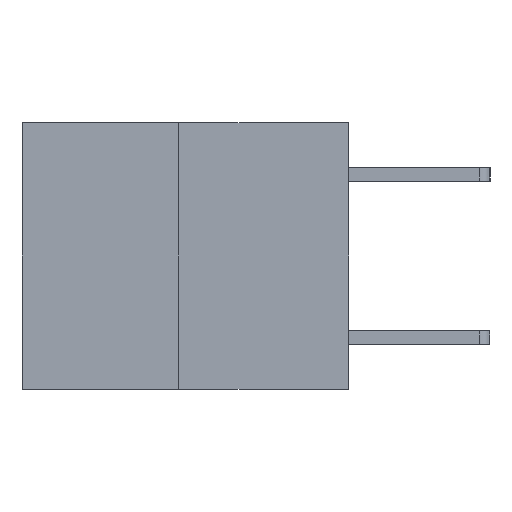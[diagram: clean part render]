
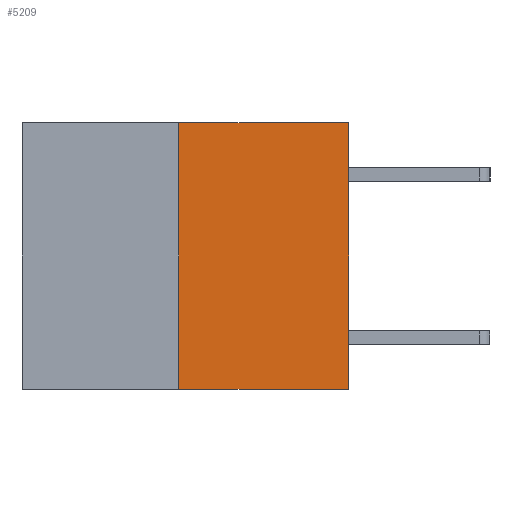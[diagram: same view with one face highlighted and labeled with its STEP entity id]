
A CAD part, left-side view. The second image highlights one B-rep face of the part: STEP entity #5209.
In plain terms, the highlighted planar face has unit normal (-1, 0, 0).
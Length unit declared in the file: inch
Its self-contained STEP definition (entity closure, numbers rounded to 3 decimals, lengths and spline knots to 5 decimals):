
#33 = ORIENTED_EDGE ( 'NONE', *, *, #299, .F. ) ;
#299 = EDGE_CURVE ( 'NONE', #6227, #8768, #3671, .T. ) ;
#565 = CARTESIAN_POINT ( 'NONE',  ( 0., 0., -0.49 ) ) ;
#566 = CARTESIAN_POINT ( 'NONE',  ( 0., 0., 0. ) ) ;
#585 = LINE ( 'NONE', #2959, #3231 ) ;
#1398 = CARTESIAN_POINT ( 'NONE',  ( 0., 0.6, 0. ) ) ;
#1475 = PLANE ( 'NONE',  #5130 ) ;
#2161 = ORIENTED_EDGE ( 'NONE', *, *, #3546, .T. ) ;
#2229 = VECTOR ( 'NONE', #4312, 39.37008 ) ;
#2291 = EDGE_CURVE ( 'NONE', #8768, #4093, #4585, .T. ) ;
#2650 = DIRECTION ( 'NONE',  ( 0., 0., 1. ) ) ;
#2959 = CARTESIAN_POINT ( 'NONE',  ( 0., 0.6, -0.49 ) ) ;
#3231 = VECTOR ( 'NONE', #9017, 39.37008 ) ;
#3359 = CARTESIAN_POINT ( 'NONE',  ( 0., 0.312, -0.49 ) ) ;
#3472 = CARTESIAN_POINT ( 'NONE',  ( 0., 0., 0. ) ) ;
#3546 = EDGE_CURVE ( 'NONE', #5984, #4093, #7043, .T. ) ;
#3671 = LINE ( 'NONE', #3359, #9608 ) ;
#3707 = EDGE_CURVE ( 'NONE', #6227, #5984, #585, .T. ) ;
#4093 = VERTEX_POINT ( 'NONE', #3472 ) ;
#4312 = DIRECTION ( 'NONE',  ( 0., 0., 1. ) ) ;
#4585 = LINE ( 'NONE', #7994, #5878 ) ;
#4590 = ORIENTED_EDGE ( 'NONE', *, *, #3707, .T. ) ;
#5130 = AXIS2_PLACEMENT_3D ( 'NONE', #1398, #5977, #6602 ) ;
#5209 = ADVANCED_FACE ( 'NONE', ( #9283 ), #1475, .F. ) ;
#5878 = VECTOR ( 'NONE', #8029, 39.37008 ) ;
#5973 = ORIENTED_EDGE ( 'NONE', *, *, #2291, .F. ) ;
#5977 = DIRECTION ( 'NONE',  ( 1., 0., 0. ) ) ;
#5984 = VERTEX_POINT ( 'NONE', #565 ) ;
#6147 = CARTESIAN_POINT ( 'NONE',  ( 0., 0.312, 0. ) ) ;
#6227 = VERTEX_POINT ( 'NONE', #8909 ) ;
#6602 = DIRECTION ( 'NONE',  ( 0., 0., -1. ) ) ;
#7043 = LINE ( 'NONE', #566, #2229 ) ;
#7994 = CARTESIAN_POINT ( 'NONE',  ( 0., 0.6, 0. ) ) ;
#8029 = DIRECTION ( 'NONE',  ( 0., -1., 0. ) ) ;
#8768 = VERTEX_POINT ( 'NONE', #6147 ) ;
#8909 = CARTESIAN_POINT ( 'NONE',  ( 0., 0.312, -0.49 ) ) ;
#9017 = DIRECTION ( 'NONE',  ( 0., -1., 0. ) ) ;
#9283 = FACE_OUTER_BOUND ( 'NONE', #9612, .T. ) ;
#9608 = VECTOR ( 'NONE', #2650, 39.37008 ) ;
#9612 = EDGE_LOOP ( 'NONE', ( #33, #4590, #2161, #5973 ) ) ;
